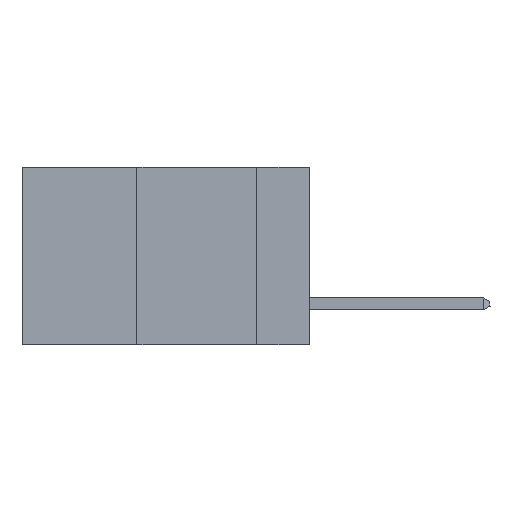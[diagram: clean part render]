
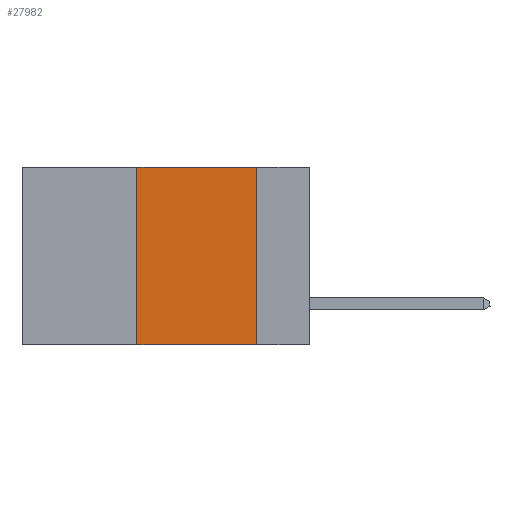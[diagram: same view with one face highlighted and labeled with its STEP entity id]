
A CAD part, left-side view. The second image highlights one B-rep face of the part: STEP entity #27982.
In plain terms, the highlighted planar face has unit normal (-1, 0, 0).
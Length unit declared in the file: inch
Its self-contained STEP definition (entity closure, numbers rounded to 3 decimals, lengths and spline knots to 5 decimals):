
#11 = ORIENTED_EDGE ( 'NONE', *, *, #22825, .T. ) ;
#613 = CARTESIAN_POINT ( 'NONE',  ( 0., 0.36, -0.37 ) ) ;
#2516 = EDGE_CURVE ( 'NONE', #26450, #28974, #23528, .T. ) ;
#3465 = LINE ( 'NONE', #16400, #5516 ) ;
#4342 = ORIENTED_EDGE ( 'NONE', *, *, #15604, .F. ) ;
#5516 = VECTOR ( 'NONE', #24255, 39.37008 ) ;
#6621 = PLANE ( 'NONE',  #10953 ) ;
#8206 = FACE_OUTER_BOUND ( 'NONE', #11748, .T. ) ;
#8404 = VERTEX_POINT ( 'NONE', #14592 ) ;
#9345 = ORIENTED_EDGE ( 'NONE', *, *, #2516, .F. ) ;
#9474 = VECTOR ( 'NONE', #22118, 39.37008 ) ;
#10953 = AXIS2_PLACEMENT_3D ( 'NONE', #27270, #30546, #19445 ) ;
#11748 = EDGE_LOOP ( 'NONE', ( #9345, #14298, #4342, #11 ) ) ;
#11922 = EDGE_CURVE ( 'NONE', #8404, #26450, #3465, .T. ) ;
#14298 = ORIENTED_EDGE ( 'NONE', *, *, #11922, .F. ) ;
#14592 = CARTESIAN_POINT ( 'NONE',  ( 0., 0.36, 0. ) ) ;
#15604 = EDGE_CURVE ( 'NONE', #18870, #8404, #30173, .T. ) ;
#16400 = CARTESIAN_POINT ( 'NONE',  ( 0., 0.6, 0. ) ) ;
#16638 = VECTOR ( 'NONE', #31973, 39.37008 ) ;
#16673 = CARTESIAN_POINT ( 'NONE',  ( 0., 0.11, 0. ) ) ;
#18169 = DIRECTION ( 'NONE',  ( 0., -1., 0. ) ) ;
#18870 = VERTEX_POINT ( 'NONE', #613 ) ;
#19445 = DIRECTION ( 'NONE',  ( 0., 0., -1. ) ) ;
#19592 = CARTESIAN_POINT ( 'NONE',  ( 0., 0.11, -0.37 ) ) ;
#21495 = VECTOR ( 'NONE', #18169, 39.37008 ) ;
#22118 = DIRECTION ( 'NONE',  ( 0., 0., 1. ) ) ;
#22740 = LINE ( 'NONE', #33588, #21495 ) ;
#22825 = EDGE_CURVE ( 'NONE', #18870, #28974, #22740, .T. ) ;
#23528 = LINE ( 'NONE', #16673, #16638 ) ;
#24255 = DIRECTION ( 'NONE',  ( 0., -1., 0. ) ) ;
#24805 = CARTESIAN_POINT ( 'NONE',  ( 0., 0.11, 0. ) ) ;
#26450 = VERTEX_POINT ( 'NONE', #24805 ) ;
#27242 = CARTESIAN_POINT ( 'NONE',  ( 0., 0.36, 0. ) ) ;
#27270 = CARTESIAN_POINT ( 'NONE',  ( 0., 0.6, 0. ) ) ;
#27982 = ADVANCED_FACE ( 'NONE', ( #8206 ), #6621, .F. ) ;
#28974 = VERTEX_POINT ( 'NONE', #19592 ) ;
#30173 = LINE ( 'NONE', #27242, #9474 ) ;
#30546 = DIRECTION ( 'NONE',  ( 1., 0., 0. ) ) ;
#31973 = DIRECTION ( 'NONE',  ( 0., 0., -1. ) ) ;
#33588 = CARTESIAN_POINT ( 'NONE',  ( 0., 0.6, -0.37 ) ) ;
